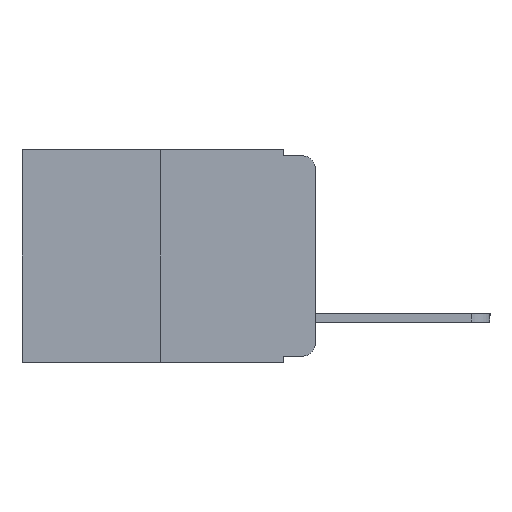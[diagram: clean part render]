
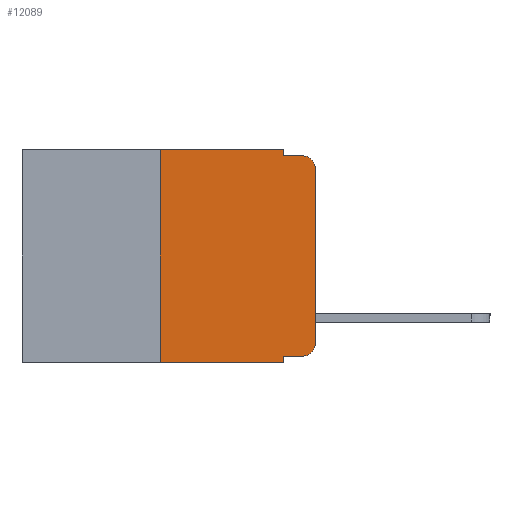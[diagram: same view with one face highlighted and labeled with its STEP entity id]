
A CAD part, left-side view. The second image highlights one B-rep face of the part: STEP entity #12089.
In plain terms, the highlighted planar face has unit normal (-1, 0, 0).
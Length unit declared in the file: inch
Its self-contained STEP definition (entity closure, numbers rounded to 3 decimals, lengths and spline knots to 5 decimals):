
#68 = DIRECTION ( 'NONE',  ( 0., 0., 1. ) ) ;
#196 = EDGE_CURVE ( 'NONE', #14934, #16019, #19331, .T. ) ;
#462 = CARTESIAN_POINT ( 'NONE',  ( 0., 0.051, 0. ) ) ;
#722 = DIRECTION ( 'NONE',  ( 1., 0., 0. ) ) ;
#1032 = VERTEX_POINT ( 'NONE', #17271 ) ;
#1435 = VECTOR ( 'NONE', #15572, 39.37008 ) ;
#2622 = ORIENTED_EDGE ( 'NONE', *, *, #11654, .F. ) ;
#2628 = VECTOR ( 'NONE', #15051, 39.37008 ) ;
#2801 = CARTESIAN_POINT ( 'NONE',  ( 0., 0.473, 0. ) ) ;
#2865 = CARTESIAN_POINT ( 'NONE',  ( 0., 0.25, 0. ) ) ;
#3383 = CARTESIAN_POINT ( 'NONE',  ( 0., 0.051, 0. ) ) ;
#3405 = AXIS2_PLACEMENT_3D ( 'NONE', #11905, #722, #13710 ) ;
#3511 = LINE ( 'NONE', #2801, #13275 ) ;
#3904 = CARTESIAN_POINT ( 'NONE',  ( 0., 0.02, -0.333 ) ) ;
#3936 = EDGE_CURVE ( 'NONE', #11193, #7436, #20791, .T. ) ;
#4284 = CARTESIAN_POINT ( 'NONE',  ( 0., 0.051, -0.01 ) ) ;
#4429 = CIRCLE ( 'NONE', #15030, 0.02 ) ;
#5194 = CARTESIAN_POINT ( 'NONE',  ( 0., 0.051, -0.343 ) ) ;
#5208 = VECTOR ( 'NONE', #17015, 39.37008 ) ;
#5400 = ORIENTED_EDGE ( 'NONE', *, *, #14036, .T. ) ;
#5581 = ORIENTED_EDGE ( 'NONE', *, *, #196, .F. ) ;
#5620 = ORIENTED_EDGE ( 'NONE', *, *, #9599, .F. ) ;
#6152 = CARTESIAN_POINT ( 'NONE',  ( 0., 0.051, -0.01 ) ) ;
#6338 = DIRECTION ( 'NONE',  ( 0., 0., -1. ) ) ;
#6542 = CARTESIAN_POINT ( 'NONE',  ( 0., 0.25, 0. ) ) ;
#6848 = CARTESIAN_POINT ( 'NONE',  ( 0., 0.02, -0.313 ) ) ;
#6982 = CARTESIAN_POINT ( 'NONE',  ( 0., 0.051, 0. ) ) ;
#7200 = CARTESIAN_POINT ( 'NONE',  ( 0., 0.473, -0.343 ) ) ;
#7425 = LINE ( 'NONE', #7200, #16567 ) ;
#7436 = VERTEX_POINT ( 'NONE', #5194 ) ;
#7507 = EDGE_CURVE ( 'NONE', #1032, #7436, #7425, .T. ) ;
#8293 = DIRECTION ( 'NONE',  ( -1., 0., 0. ) ) ;
#8487 = ORIENTED_EDGE ( 'NONE', *, *, #9021, .T. ) ;
#8720 = DIRECTION ( 'NONE',  ( 0., 0., -1. ) ) ;
#8791 = ORIENTED_EDGE ( 'NONE', *, *, #7507, .T. ) ;
#9021 = EDGE_CURVE ( 'NONE', #12929, #16019, #4429, .T. ) ;
#9072 = DIRECTION ( 'NONE',  ( 0., -1., 0. ) ) ;
#9240 = ORIENTED_EDGE ( 'NONE', *, *, #3936, .F. ) ;
#9599 = EDGE_CURVE ( 'NONE', #19379, #19604, #3511, .T. ) ;
#9676 = EDGE_CURVE ( 'NONE', #12546, #11391, #20197, .T. ) ;
#9760 = ORIENTED_EDGE ( 'NONE', *, *, #14522, .F. ) ;
#11135 = ORIENTED_EDGE ( 'NONE', *, *, #19086, .T. ) ;
#11193 = VERTEX_POINT ( 'NONE', #18054 ) ;
#11338 = LINE ( 'NONE', #6542, #1435 ) ;
#11391 = VERTEX_POINT ( 'NONE', #15025 ) ;
#11520 = CARTESIAN_POINT ( 'NONE',  ( 0., 0.051, -0.333 ) ) ;
#11654 = EDGE_CURVE ( 'NONE', #1032, #19379, #11338, .T. ) ;
#11905 = CARTESIAN_POINT ( 'NONE',  ( 0., 0.473, 0. ) ) ;
#12089 = ADVANCED_FACE ( 'NONE', ( #14407 ), #15453, .F. ) ;
#12546 = VERTEX_POINT ( 'NONE', #3904 ) ;
#12798 = CARTESIAN_POINT ( 'NONE',  ( 0., 0.02, -0.01 ) ) ;
#12929 = VERTEX_POINT ( 'NONE', #15734 ) ;
#12940 = LINE ( 'NONE', #11520, #2628 ) ;
#13275 = VECTOR ( 'NONE', #13800, 39.37008 ) ;
#13559 = ORIENTED_EDGE ( 'NONE', *, *, #9676, .T. ) ;
#13710 = DIRECTION ( 'NONE',  ( 0., 0., -1. ) ) ;
#13726 = LINE ( 'NONE', #21489, #17838 ) ;
#13800 = DIRECTION ( 'NONE',  ( 0., -1., 0. ) ) ;
#14036 = EDGE_CURVE ( 'NONE', #11391, #12929, #13726, .T. ) ;
#14407 = FACE_OUTER_BOUND ( 'NONE', #18459, .T. ) ;
#14522 = EDGE_CURVE ( 'NONE', #19604, #14934, #19899, .T. ) ;
#14586 = AXIS2_PLACEMENT_3D ( 'NONE', #6848, #19258, #8720 ) ;
#14934 = VERTEX_POINT ( 'NONE', #6152 ) ;
#15025 = CARTESIAN_POINT ( 'NONE',  ( 0., 0., -0.313 ) ) ;
#15030 = AXIS2_PLACEMENT_3D ( 'NONE', #18940, #8293, #20491 ) ;
#15051 = DIRECTION ( 'NONE',  ( 0., -1., 0. ) ) ;
#15453 = PLANE ( 'NONE',  #3405 ) ;
#15572 = DIRECTION ( 'NONE',  ( 0., 0., 1. ) ) ;
#15734 = CARTESIAN_POINT ( 'NONE',  ( 0., 0., -0.03 ) ) ;
#16019 = VERTEX_POINT ( 'NONE', #12798 ) ;
#16537 = VECTOR ( 'NONE', #6338, 39.37008 ) ;
#16567 = VECTOR ( 'NONE', #9072, 39.37008 ) ;
#17015 = DIRECTION ( 'NONE',  ( 0., 0., -1. ) ) ;
#17271 = CARTESIAN_POINT ( 'NONE',  ( 0., 0.25, -0.343 ) ) ;
#17838 = VECTOR ( 'NONE', #68, 39.37008 ) ;
#18054 = CARTESIAN_POINT ( 'NONE',  ( 0., 0.051, -0.333 ) ) ;
#18364 = DIRECTION ( 'NONE',  ( 0., -1., 0. ) ) ;
#18459 = EDGE_LOOP ( 'NONE', ( #5400, #8487, #5581, #9760, #5620, #2622, #8791, #9240, #11135, #13559 ) ) ;
#18940 = CARTESIAN_POINT ( 'NONE',  ( 0., 0.02, -0.03 ) ) ;
#19086 = EDGE_CURVE ( 'NONE', #11193, #12546, #12940, .T. ) ;
#19258 = DIRECTION ( 'NONE',  ( -1., 0., 0. ) ) ;
#19331 = LINE ( 'NONE', #4284, #22518 ) ;
#19379 = VERTEX_POINT ( 'NONE', #2865 ) ;
#19604 = VERTEX_POINT ( 'NONE', #6982 ) ;
#19899 = LINE ( 'NONE', #462, #5208 ) ;
#20197 = CIRCLE ( 'NONE', #14586, 0.02 ) ;
#20491 = DIRECTION ( 'NONE',  ( 0., 0., -1. ) ) ;
#20791 = LINE ( 'NONE', #3383, #16537 ) ;
#21489 = CARTESIAN_POINT ( 'NONE',  ( 0., 0., 0. ) ) ;
#22518 = VECTOR ( 'NONE', #18364, 39.37008 ) ;
